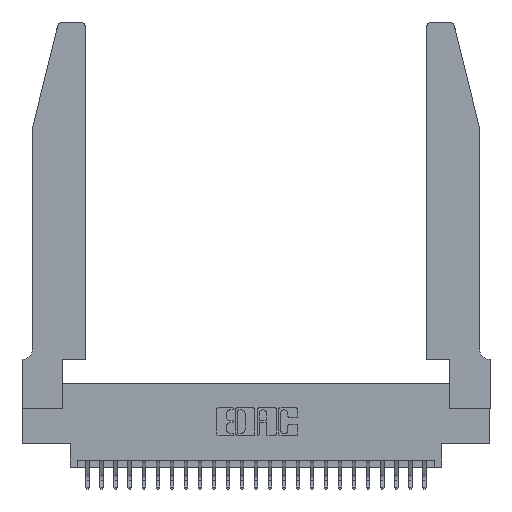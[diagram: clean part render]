
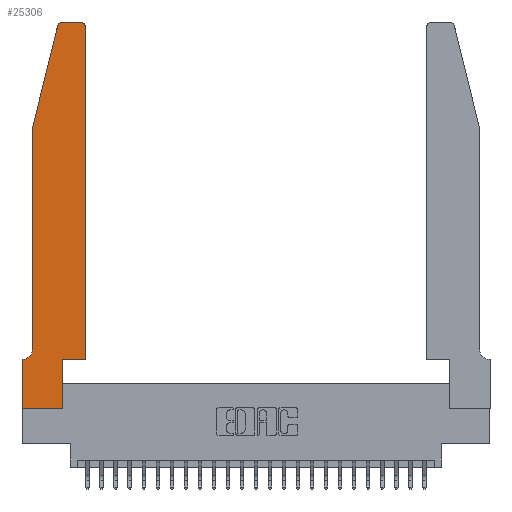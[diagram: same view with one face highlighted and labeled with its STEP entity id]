
A CAD part, top view. The second image highlights one B-rep face of the part: STEP entity #25306.
In plain terms, the highlighted planar face has unit normal (0, 0, 1).
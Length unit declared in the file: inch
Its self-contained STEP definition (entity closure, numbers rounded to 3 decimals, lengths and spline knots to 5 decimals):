
#11 = VECTOR ( 'NONE', #11764, 39.37008 ) ;
#43 = DIRECTION ( 'NONE',  ( 1., 0., 0. ) ) ;
#460 = VECTOR ( 'NONE', #8726, 39.37008 ) ;
#1127 = EDGE_LOOP ( 'NONE', ( #4548, #12040, #5875, #12748, #20885, #22409, #26920, #17766, #26105, #6116, #9721, #13203 ) ) ;
#1307 = VERTEX_POINT ( 'NONE', #10090 ) ;
#2068 = DIRECTION ( 'NONE',  ( 0., 0., 1. ) ) ;
#2521 = VECTOR ( 'NONE', #4084, 39.37008 ) ;
#2529 = EDGE_CURVE ( 'NONE', #10185, #6808, #17865, .T. ) ;
#2702 = CARTESIAN_POINT ( 'NONE',  ( 0.25487, 2.72718, 0.37 ) ) ;
#3785 = LINE ( 'NONE', #10937, #24308 ) ;
#4084 = DIRECTION ( 'NONE',  ( -1., 0., 0. ) ) ;
#4506 = VERTEX_POINT ( 'NONE', #6332 ) ;
#4548 = ORIENTED_EDGE ( 'NONE', *, *, #19845, .T. ) ;
#4582 = CARTESIAN_POINT ( 'NONE',  ( 0.0755, 2., 0.37 ) ) ;
#4747 = LINE ( 'NONE', #22992, #460 ) ;
#4752 = VERTEX_POINT ( 'NONE', #2702 ) ;
#4992 = CARTESIAN_POINT ( 'NONE',  ( 0.4505, 0.35, 0.37 ) ) ;
#5313 = CARTESIAN_POINT ( 'NONE',  ( 0., 0., 0.37 ) ) ;
#5336 = CARTESIAN_POINT ( 'NONE',  ( 0.284, 2.72, 0.37 ) ) ;
#5610 = LINE ( 'NONE', #15959, #11 ) ;
#5875 = ORIENTED_EDGE ( 'NONE', *, *, #26755, .T. ) ;
#6116 = ORIENTED_EDGE ( 'NONE', *, *, #15792, .T. ) ;
#6332 = CARTESIAN_POINT ( 'NONE',  ( 0.4205, 2.75, 0.37 ) ) ;
#6514 = CARTESIAN_POINT ( 'NONE',  ( 0.4505, 2.72, 0.37 ) ) ;
#6766 = CARTESIAN_POINT ( 'NONE',  ( 0.2605, 2.75, 0.37 ) ) ;
#6808 = VERTEX_POINT ( 'NONE', #16045 ) ;
#7099 = CIRCLE ( 'NONE', #15201, 0.03 ) ;
#7368 = DIRECTION ( 'NONE',  ( -1., 0., 0. ) ) ;
#7387 = AXIS2_PLACEMENT_3D ( 'NONE', #25764, #21568, #7368 ) ;
#7419 = EDGE_CURVE ( 'NONE', #26155, #21784, #5610, .T. ) ;
#7512 = VECTOR ( 'NONE', #25327, 39.37008 ) ;
#7717 = CIRCLE ( 'NONE', #7387, 0.07 ) ;
#7906 = VERTEX_POINT ( 'NONE', #6514 ) ;
#8726 = DIRECTION ( 'NONE',  ( 1., 0., 0. ) ) ;
#8744 = EDGE_CURVE ( 'NONE', #26239, #15385, #14682, .T. ) ;
#8882 = DIRECTION ( 'NONE',  ( -1., 0., 0. ) ) ;
#9000 = CARTESIAN_POINT ( 'NONE',  ( 0.0755, 2., 0.37 ) ) ;
#9721 = ORIENTED_EDGE ( 'NONE', *, *, #20171, .T. ) ;
#10090 = CARTESIAN_POINT ( 'NONE',  ( 0.4505, 0.35, 0.37 ) ) ;
#10185 = VERTEX_POINT ( 'NONE', #22762 ) ;
#10937 = CARTESIAN_POINT ( 'NONE',  ( 0., 0., 0.37 ) ) ;
#11764 = DIRECTION ( 'NONE',  ( 0., -1., 0. ) ) ;
#12040 = ORIENTED_EDGE ( 'NONE', *, *, #13228, .T. ) ;
#12748 = ORIENTED_EDGE ( 'NONE', *, *, #7419, .T. ) ;
#13203 = ORIENTED_EDGE ( 'NONE', *, *, #21311, .T. ) ;
#13228 = EDGE_CURVE ( 'NONE', #19039, #4752, #7099, .T. ) ;
#13584 = VECTOR ( 'NONE', #21234, 39.37008 ) ;
#13680 = VECTOR ( 'NONE', #8882, 39.37008 ) ;
#13722 = DIRECTION ( 'NONE',  ( 0., -1., 0. ) ) ;
#14682 = LINE ( 'NONE', #24870, #7512 ) ;
#14897 = DIRECTION ( 'NONE',  ( 1., 0., 0. ) ) ;
#15201 = AXIS2_PLACEMENT_3D ( 'NONE', #5336, #17887, #18082 ) ;
#15385 = VERTEX_POINT ( 'NONE', #26129 ) ;
#15651 = PLANE ( 'NONE',  #21731 ) ;
#15792 = EDGE_CURVE ( 'NONE', #15385, #1307, #4747, .T. ) ;
#15820 = DIRECTION ( 'NONE',  ( 0., 0., 1. ) ) ;
#15959 = CARTESIAN_POINT ( 'NONE',  ( 0.0755, 2., 0.37 ) ) ;
#16045 = CARTESIAN_POINT ( 'NONE',  ( 0., 0.35, 0.37 ) ) ;
#17496 = CARTESIAN_POINT ( 'NONE',  ( 0., 0., 0.37 ) ) ;
#17766 = ORIENTED_EDGE ( 'NONE', *, *, #26685, .T. ) ;
#17865 = LINE ( 'NONE', #27030, #2521 ) ;
#17887 = DIRECTION ( 'NONE',  ( 0., 0., 1. ) ) ;
#18082 = DIRECTION ( 'NONE',  ( 1., 0., 0. ) ) ;
#18561 = VECTOR ( 'NONE', #13722, 39.37008 ) ;
#18883 = LINE ( 'NONE', #4992, #22453 ) ;
#19039 = VERTEX_POINT ( 'NONE', #23175 ) ;
#19101 = LINE ( 'NONE', #4582, #13584 ) ;
#19188 = LINE ( 'NONE', #6766, #13680 ) ;
#19845 = EDGE_CURVE ( 'NONE', #4506, #19039, #19188, .T. ) ;
#19978 = VERTEX_POINT ( 'NONE', #17496 ) ;
#20171 = EDGE_CURVE ( 'NONE', #1307, #7906, #18883, .T. ) ;
#20885 = ORIENTED_EDGE ( 'NONE', *, *, #22074, .T. ) ;
#21041 = CARTESIAN_POINT ( 'NONE',  ( 0.4205, 2.72, 0.37 ) ) ;
#21234 = DIRECTION ( 'NONE',  ( -0.239, -0.971, 0. ) ) ;
#21311 = EDGE_CURVE ( 'NONE', #7906, #4506, #22067, .T. ) ;
#21568 = DIRECTION ( 'NONE',  ( 0., 0., -1. ) ) ;
#21657 = DIRECTION ( 'NONE',  ( 0., 1., 0. ) ) ;
#21731 = AXIS2_PLACEMENT_3D ( 'NONE', #26113, #15820, #21826 ) ;
#21784 = VERTEX_POINT ( 'NONE', #26766 ) ;
#21826 = DIRECTION ( 'NONE',  ( 1., 0., 0. ) ) ;
#22067 = CIRCLE ( 'NONE', #23243, 0.03 ) ;
#22074 = EDGE_CURVE ( 'NONE', #21784, #10185, #7717, .T. ) ;
#22409 = ORIENTED_EDGE ( 'NONE', *, *, #2529, .T. ) ;
#22453 = VECTOR ( 'NONE', #21657, 39.37008 ) ;
#22762 = CARTESIAN_POINT ( 'NONE',  ( 0.0055, 0.35, 0.37 ) ) ;
#22992 = CARTESIAN_POINT ( 'NONE',  ( 0.4505, 0.35, 0.37 ) ) ;
#23106 = LINE ( 'NONE', #5313, #18561 ) ;
#23175 = CARTESIAN_POINT ( 'NONE',  ( 0.284, 2.75, 0.37 ) ) ;
#23243 = AXIS2_PLACEMENT_3D ( 'NONE', #21041, #2068, #43 ) ;
#23627 = CARTESIAN_POINT ( 'NONE',  ( 0.2865, 0., 0.37 ) ) ;
#24102 = EDGE_CURVE ( 'NONE', #6808, #19978, #23106, .T. ) ;
#24308 = VECTOR ( 'NONE', #14897, 39.37008 ) ;
#24870 = CARTESIAN_POINT ( 'NONE',  ( 0.2865, 0.35, 0.37 ) ) ;
#25306 = ADVANCED_FACE ( 'NONE', ( #25724 ), #15651, .T. ) ;
#25327 = DIRECTION ( 'NONE',  ( 0., 1., 0. ) ) ;
#25724 = FACE_OUTER_BOUND ( 'NONE', #1127, .T. ) ;
#25764 = CARTESIAN_POINT ( 'NONE',  ( 0.0055, 0.42, 0.37 ) ) ;
#26105 = ORIENTED_EDGE ( 'NONE', *, *, #8744, .T. ) ;
#26113 = CARTESIAN_POINT ( 'NONE',  ( 0., 0.35, 0.37 ) ) ;
#26129 = CARTESIAN_POINT ( 'NONE',  ( 0.2865, 0.35, 0.37 ) ) ;
#26155 = VERTEX_POINT ( 'NONE', #9000 ) ;
#26239 = VERTEX_POINT ( 'NONE', #23627 ) ;
#26685 = EDGE_CURVE ( 'NONE', #19978, #26239, #3785, .T. ) ;
#26755 = EDGE_CURVE ( 'NONE', #4752, #26155, #19101, .T. ) ;
#26766 = CARTESIAN_POINT ( 'NONE',  ( 0.0755, 0.42, 0.37 ) ) ;
#26920 = ORIENTED_EDGE ( 'NONE', *, *, #24102, .T. ) ;
#27030 = CARTESIAN_POINT ( 'NONE',  ( 0.0755, 0.35, 0.37 ) ) ;
